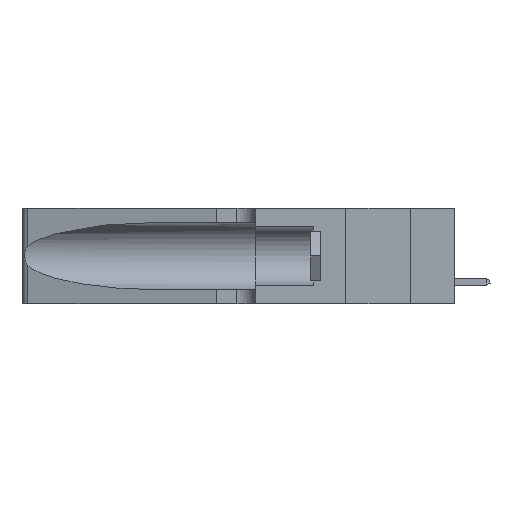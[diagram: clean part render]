
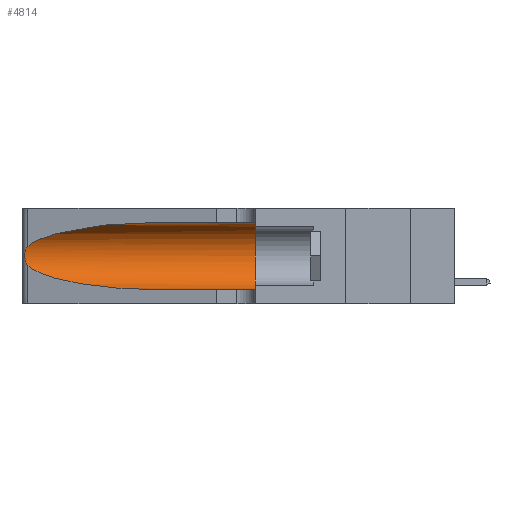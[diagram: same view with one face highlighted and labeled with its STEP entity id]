
A CAD part, left-side view. The second image highlights one B-rep face of the part: STEP entity #4814.
In plain terms, the highlighted cylindrical face has radius 3.308 mm (diameter 6.617 mm), a partial arc.
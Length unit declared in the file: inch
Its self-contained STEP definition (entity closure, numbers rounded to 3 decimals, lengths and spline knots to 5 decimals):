
#100 = EDGE_LOOP ( 'NONE', ( #31168, #18167, #2252, #26772, #7129, #13239 ) ) ;
#249 = CARTESIAN_POINT ( 'NONE',  ( 0.26075, 1.23896, 0.178 ) ) ;
#596 = VERTEX_POINT ( 'NONE', #32067 ) ;
#818 = CARTESIAN_POINT ( 'NONE',  ( 0.18966, 0.96281, 0.05475 ) ) ;
#1022 = DIRECTION ( 'NONE',  ( 0., 1., 0. ) ) ;
#1153 = DIRECTION ( 'NONE',  ( 0., -1., 0. ) ) ;
#2252 = ORIENTED_EDGE ( 'NONE', *, *, #36732, .T. ) ;
#3150 = CARTESIAN_POINT ( 'NONE',  ( 0.25639, 1.23186, 0.15144 ) ) ;
#3565 = CIRCLE ( 'NONE', #35512, 0.13025 ) ;
#3683 = CARTESIAN_POINT ( 'NONE',  ( 0.2373, 1.15595, 0.28018 ) ) ;
#3792 = CARTESIAN_POINT ( 'NONE',  ( 0.1305, 0.35, 0.31525 ) ) ;
#4578 = CARTESIAN_POINT ( 'NONE',  ( 0.1305, 0.35, 0.185 ) ) ;
#4814 = ADVANCED_FACE ( 'NONE', ( #16704 ), #12837, .F. ) ;
#5015 = CARTESIAN_POINT ( 'NONE',  ( 0.26017, 1.23833, 0.17102 ) ) ;
#6320 = CARTESIAN_POINT ( 'NONE',  ( 0.1305, 0.72297, 0.05475 ) ) ;
#7129 = ORIENTED_EDGE ( 'NONE', *, *, #21017, .F. ) ;
#7807 =( BOUNDED_CURVE ( )  B_SPLINE_CURVE ( 3, ( #31405, #37654, #3683, #38461 ),
 .UNSPECIFIED., .F., .F. ) 
 B_SPLINE_CURVE_WITH_KNOTS ( ( 4, 4 ),
 ( 1.5708, 2.84003 ),
 .UNSPECIFIED. ) 
 CURVE ( )  GEOMETRIC_REPRESENTATION_ITEM ( )  RATIONAL_B_SPLINE_CURVE ( ( 1., 0.87, 0.87, 1. ) ) 
 REPRESENTATION_ITEM ( '' )  );
#9195 = VERTEX_POINT ( 'NONE', #17375 ) ;
#9933 = CARTESIAN_POINT ( 'NONE',  ( 0.25555, 1.22993, 0.14849 ) ) ;
#9996 = CARTESIAN_POINT ( 'NONE',  ( 0.26075, 1.23896, 0.19203 ) ) ;
#10952 = CARTESIAN_POINT ( 'NONE',  ( 0.1305, 1.61858, 0.185 ) ) ;
#11621 = EDGE_CURVE ( 'NONE', #35407, #11976, #27134, .T. ) ;
#11976 = VERTEX_POINT ( 'NONE', #3792 ) ;
#11991 = CARTESIAN_POINT ( 'NONE',  ( 0.2373, 1.15595, 0.08982 ) ) ;
#12235 = CARTESIAN_POINT ( 'NONE',  ( 0.25854, 1.2359, 0.20912 ) ) ;
#12837 = CYLINDRICAL_SURFACE ( 'NONE', #36766, 0.13025 ) ;
#12956 = CARTESIAN_POINT ( 'NONE',  ( 0.1305, 1.61858, 0.05475 ) ) ;
#13239 = ORIENTED_EDGE ( 'NONE', *, *, #11621, .F. ) ;
#13514 = DIRECTION ( 'NONE',  ( 0., 0., 1. ) ) ;
#14182 = CARTESIAN_POINT ( 'NONE',  ( 0.25487, 1.22718, 0.14631 ) ) ;
#14261 = EDGE_CURVE ( 'NONE', #35407, #9195, #7807, .T. ) ;
#15200 = CARTESIAN_POINT ( 'NONE',  ( 0.25639, 1.23184, 0.21858 ) ) ;
#15712 = CARTESIAN_POINT ( 'NONE',  ( 0.26018, 1.23835, 0.19895 ) ) ;
#16704 = FACE_OUTER_BOUND ( 'NONE', #100, .T. ) ;
#17375 = CARTESIAN_POINT ( 'NONE',  ( 0.25487, 1.22718, 0.22369 ) ) ;
#17462 = DIRECTION ( 'NONE',  ( 0., 0., -1. ) ) ;
#18000 =( BOUNDED_CURVE ( )  B_SPLINE_CURVE ( 3, ( #30487, #11991, #818, #22452 ),
 .UNSPECIFIED., .F., .T. ) 
 B_SPLINE_CURVE_WITH_KNOTS ( ( 4, 4 ),
 ( 3.44316, 4.71239 ),
 .UNSPECIFIED. ) 
 CURVE ( )  GEOMETRIC_REPRESENTATION_ITEM ( )  RATIONAL_B_SPLINE_CURVE ( ( 1., 0.87, 0.87, 1. ) ) 
 REPRESENTATION_ITEM ( '' )  );
#18167 = ORIENTED_EDGE ( 'NONE', *, *, #29279, .T. ) ;
#18299 = CARTESIAN_POINT ( 'NONE',  ( 0.25787, 1.23484, 0.2124 ) ) ;
#20252 = CARTESIAN_POINT ( 'NONE',  ( 0.1305, 1.61858, 0.31525 ) ) ;
#20473 = CARTESIAN_POINT ( 'NONE',  ( 0.25856, 1.23593, 0.16098 ) ) ;
#20981 = B_SPLINE_CURVE_WITH_KNOTS ( 'NONE', 3,
 ( #34114, #24263, #15200, #18299, #12235, #15712, #9996, #249, #5015, #20473, #22251, #3150, #9933, #14182 ),
 .UNSPECIFIED., .F., .F.,
 ( 4, 2, 2, 2, 2, 2, 4 ),
 ( 0., 0.00027, 0.00053, 0.00107, 0.0016, 0.00187, 0.00214 ),
 .UNSPECIFIED. ) ;
#21017 = EDGE_CURVE ( 'NONE', #11976, #23443, #3565, .T. ) ;
#21365 = LINE ( 'NONE', #12956, #38785 ) ;
#21699 = CARTESIAN_POINT ( 'NONE',  ( 0.1305, 0.72297, 0.31525 ) ) ;
#22251 = CARTESIAN_POINT ( 'NONE',  ( 0.25789, 1.23486, 0.15765 ) ) ;
#22452 = CARTESIAN_POINT ( 'NONE',  ( 0.1305, 0.72297, 0.05475 ) ) ;
#23425 = EDGE_CURVE ( 'NONE', #23646, #23443, #21365, .T. ) ;
#23443 = VERTEX_POINT ( 'NONE', #37981 ) ;
#23646 = VERTEX_POINT ( 'NONE', #6320 ) ;
#24263 = CARTESIAN_POINT ( 'NONE',  ( 0.25555, 1.22994, 0.2215 ) ) ;
#26612 = DIRECTION ( 'NONE',  ( 0., -1., 0. ) ) ;
#26772 = ORIENTED_EDGE ( 'NONE', *, *, #23425, .T. ) ;
#27134 = LINE ( 'NONE', #20252, #38264 ) ;
#29279 = EDGE_CURVE ( 'NONE', #9195, #596, #20981, .T. ) ;
#30487 = CARTESIAN_POINT ( 'NONE',  ( 0.25487, 1.22718, 0.14631 ) ) ;
#31168 = ORIENTED_EDGE ( 'NONE', *, *, #14261, .T. ) ;
#31405 = CARTESIAN_POINT ( 'NONE',  ( 0.1305, 0.72297, 0.31525 ) ) ;
#32067 = CARTESIAN_POINT ( 'NONE',  ( 0.25487, 1.22718, 0.14631 ) ) ;
#34114 = CARTESIAN_POINT ( 'NONE',  ( 0.25487, 1.22718, 0.22369 ) ) ;
#35407 = VERTEX_POINT ( 'NONE', #21699 ) ;
#35451 = DIRECTION ( 'NONE',  ( 0., -1., 0. ) ) ;
#35512 = AXIS2_PLACEMENT_3D ( 'NONE', #4578, #1022, #13514 ) ;
#36732 = EDGE_CURVE ( 'NONE', #596, #23646, #18000, .T. ) ;
#36766 = AXIS2_PLACEMENT_3D ( 'NONE', #10952, #35451, #17462 ) ;
#37654 = CARTESIAN_POINT ( 'NONE',  ( 0.18966, 0.96281, 0.31525 ) ) ;
#37981 = CARTESIAN_POINT ( 'NONE',  ( 0.1305, 0.35, 0.05475 ) ) ;
#38264 = VECTOR ( 'NONE', #26612, 39.37008 ) ;
#38461 = CARTESIAN_POINT ( 'NONE',  ( 0.25487, 1.22718, 0.22369 ) ) ;
#38785 = VECTOR ( 'NONE', #1153, 39.37008 ) ;
